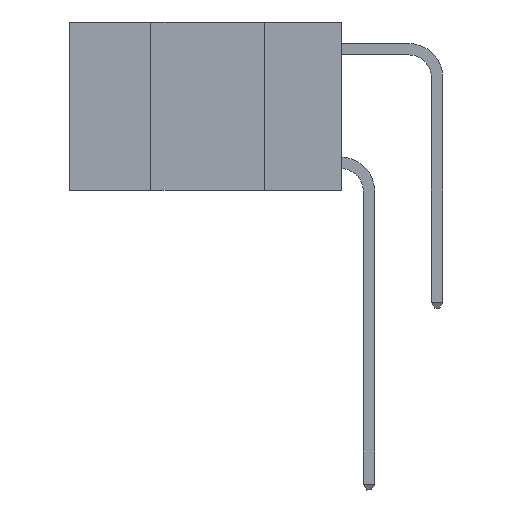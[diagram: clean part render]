
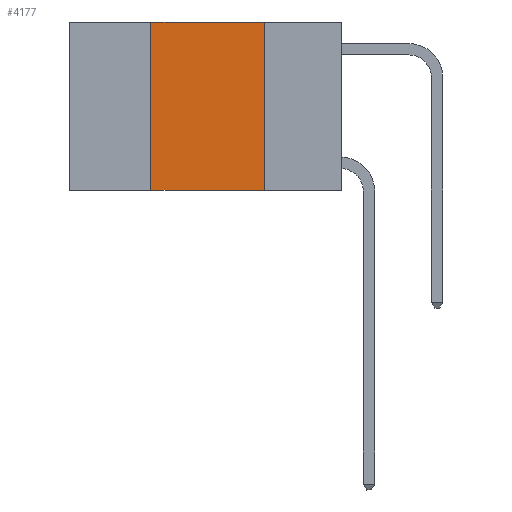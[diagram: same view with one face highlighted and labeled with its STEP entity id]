
A CAD part, left-side view. The second image highlights one B-rep face of the part: STEP entity #4177.
In plain terms, the highlighted planar face has unit normal (-1, 0, 0).
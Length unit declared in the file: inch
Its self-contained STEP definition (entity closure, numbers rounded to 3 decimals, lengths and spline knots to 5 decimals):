
#429 = EDGE_LOOP ( 'NONE', ( #4411, #9409, #12020, #9979 ) ) ;
#1217 = VERTEX_POINT ( 'NONE', #11372 ) ;
#1574 = VECTOR ( 'NONE', #9730, 39.37008 ) ;
#2099 = DIRECTION ( 'NONE',  ( 0., 0., -1. ) ) ;
#2127 = EDGE_CURVE ( 'NONE', #8735, #5819, #11473, .T. ) ;
#2737 = AXIS2_PLACEMENT_3D ( 'NONE', #4272, #10723, #6113 ) ;
#2769 = FACE_OUTER_BOUND ( 'NONE', #429, .T. ) ;
#3505 = LINE ( 'NONE', #7017, #8164 ) ;
#3569 = CARTESIAN_POINT ( 'NONE',  ( 0., 0.42, -0.37 ) ) ;
#3884 = VECTOR ( 'NONE', #2099, 39.37008 ) ;
#4177 = ADVANCED_FACE ( 'NONE', ( #2769 ), #5193, .F. ) ;
#4272 = CARTESIAN_POINT ( 'NONE',  ( 0., 0.6, 0. ) ) ;
#4411 = ORIENTED_EDGE ( 'NONE', *, *, #11108, .F. ) ;
#5193 = PLANE ( 'NONE',  #2737 ) ;
#5819 = VERTEX_POINT ( 'NONE', #8356 ) ;
#6113 = DIRECTION ( 'NONE',  ( 0., 0., -1. ) ) ;
#6318 = LINE ( 'NONE', #8659, #3884 ) ;
#7017 = CARTESIAN_POINT ( 'NONE',  ( 0., 0.42, 0. ) ) ;
#7529 = CARTESIAN_POINT ( 'NONE',  ( 0., 0.42, 0. ) ) ;
#7691 = EDGE_CURVE ( 'NONE', #8561, #8735, #3505, .T. ) ;
#7982 = EDGE_CURVE ( 'NONE', #8561, #1217, #8015, .T. ) ;
#7987 = DIRECTION ( 'NONE',  ( 0., 0., 1. ) ) ;
#8015 = LINE ( 'NONE', #11160, #9914 ) ;
#8164 = VECTOR ( 'NONE', #7987, 39.37008 ) ;
#8356 = CARTESIAN_POINT ( 'NONE',  ( 0., 0.17, 0. ) ) ;
#8561 = VERTEX_POINT ( 'NONE', #3569 ) ;
#8659 = CARTESIAN_POINT ( 'NONE',  ( 0., 0.17, 0. ) ) ;
#8735 = VERTEX_POINT ( 'NONE', #7529 ) ;
#9381 = DIRECTION ( 'NONE',  ( 0., -1., 0. ) ) ;
#9409 = ORIENTED_EDGE ( 'NONE', *, *, #2127, .F. ) ;
#9715 = CARTESIAN_POINT ( 'NONE',  ( 0., 0.6, 0. ) ) ;
#9730 = DIRECTION ( 'NONE',  ( 0., -1., 0. ) ) ;
#9914 = VECTOR ( 'NONE', #9381, 39.37008 ) ;
#9979 = ORIENTED_EDGE ( 'NONE', *, *, #7982, .T. ) ;
#10723 = DIRECTION ( 'NONE',  ( 1., 0., 0. ) ) ;
#11108 = EDGE_CURVE ( 'NONE', #5819, #1217, #6318, .T. ) ;
#11160 = CARTESIAN_POINT ( 'NONE',  ( 0., 0.6, -0.37 ) ) ;
#11372 = CARTESIAN_POINT ( 'NONE',  ( 0., 0.17, -0.37 ) ) ;
#11473 = LINE ( 'NONE', #9715, #1574 ) ;
#12020 = ORIENTED_EDGE ( 'NONE', *, *, #7691, .F. ) ;
